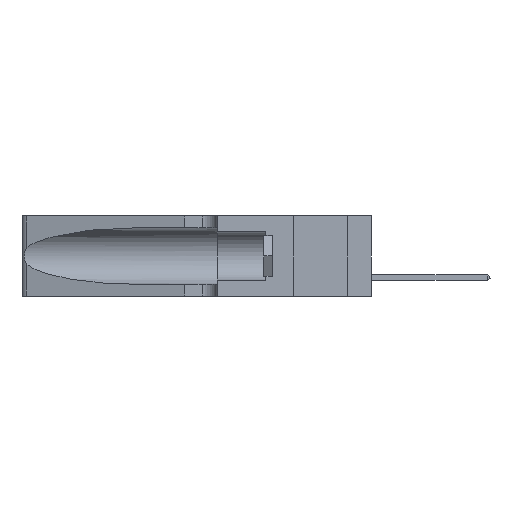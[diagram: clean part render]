
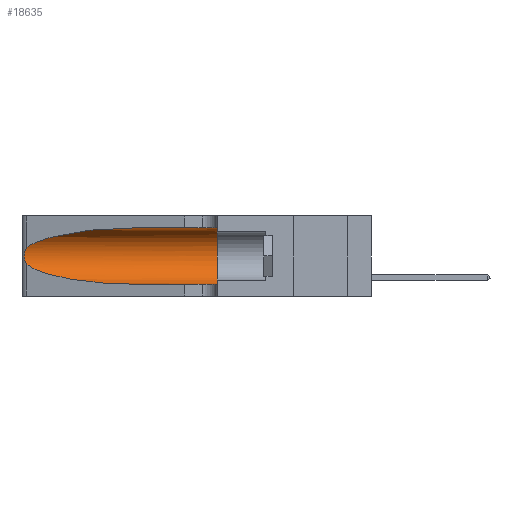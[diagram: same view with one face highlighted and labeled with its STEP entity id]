
A CAD part, left-side view. The second image highlights one B-rep face of the part: STEP entity #18635.
In plain terms, the highlighted cylindrical face has radius 3.308 mm (diameter 6.617 mm), a partial arc.
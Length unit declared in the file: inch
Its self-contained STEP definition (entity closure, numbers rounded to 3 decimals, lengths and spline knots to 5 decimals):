
#292 = DIRECTION ( 'NONE',  ( 0., 0., 1. ) ) ;
#557 = CARTESIAN_POINT ( 'NONE',  ( 0.26075, 1.23896, 0.19203 ) ) ;
#892 = DIRECTION ( 'NONE',  ( 0., -1., 0. ) ) ;
#2147 = VERTEX_POINT ( 'NONE', #2160 ) ;
#2160 = CARTESIAN_POINT ( 'NONE',  ( 0.1305, 0.35, 0.31525 ) ) ;
#2816 = VERTEX_POINT ( 'NONE', #16164 ) ;
#2926 = CIRCLE ( 'NONE', #32977, 0.13025 ) ;
#3227 = CARTESIAN_POINT ( 'NONE',  ( 0.25487, 1.22718, 0.14631 ) ) ;
#3683 = DIRECTION ( 'NONE',  ( 0., 1., 0. ) ) ;
#3934 = CARTESIAN_POINT ( 'NONE',  ( 0.26018, 1.23835, 0.19895 ) ) ;
#4049 = LINE ( 'NONE', #35554, #8653 ) ;
#6764 = ORIENTED_EDGE ( 'NONE', *, *, #40059, .F. ) ;
#6802 = B_SPLINE_CURVE_WITH_KNOTS ( 'NONE', 3,
 ( #33752, #18810, #18976, #15438, #41116, #3934, #557, #19125, #15267, #15605, #7940, #11276, #44798, #44950 ),
 .UNSPECIFIED., .F., .F.,
 ( 4, 2, 2, 2, 2, 2, 4 ),
 ( 0., 0.00027, 0.00053, 0.00107, 0.0016, 0.00187, 0.00214 ),
 .UNSPECIFIED. ) ;
#7940 = CARTESIAN_POINT ( 'NONE',  ( 0.25789, 1.23486, 0.15765 ) ) ;
#7962 = CARTESIAN_POINT ( 'NONE',  ( 0.1305, 1.61858, 0.31525 ) ) ;
#8653 = VECTOR ( 'NONE', #16770, 39.37008 ) ;
#11044 = CARTESIAN_POINT ( 'NONE',  ( 0.2373, 1.15595, 0.08982 ) ) ;
#11276 = CARTESIAN_POINT ( 'NONE',  ( 0.25639, 1.23186, 0.15144 ) ) ;
#13422 = DIRECTION ( 'NONE',  ( 0., 0., -1. ) ) ;
#14965 = CARTESIAN_POINT ( 'NONE',  ( 0.25487, 1.22718, 0.22369 ) ) ;
#15267 = CARTESIAN_POINT ( 'NONE',  ( 0.26017, 1.23833, 0.17102 ) ) ;
#15311 =( BOUNDED_CURVE ( )  B_SPLINE_CURVE ( 3, ( #25751, #32349, #43531, #14965 ),
 .UNSPECIFIED., .F., .F. ) 
 B_SPLINE_CURVE_WITH_KNOTS ( ( 4, 4 ),
 ( 1.5708, 2.84003 ),
 .UNSPECIFIED. ) 
 CURVE ( )  GEOMETRIC_REPRESENTATION_ITEM ( )  RATIONAL_B_SPLINE_CURVE ( ( 1., 0.87, 0.87, 1. ) ) 
 REPRESENTATION_ITEM ( '' )  );
#15438 = CARTESIAN_POINT ( 'NONE',  ( 0.25787, 1.23484, 0.2124 ) ) ;
#15444 = VECTOR ( 'NONE', #892, 39.37008 ) ;
#15605 = CARTESIAN_POINT ( 'NONE',  ( 0.25856, 1.23593, 0.16098 ) ) ;
#16164 = CARTESIAN_POINT ( 'NONE',  ( 0.1305, 0.72297, 0.05475 ) ) ;
#16770 = DIRECTION ( 'NONE',  ( 0., -1., 0. ) ) ;
#17588 = VERTEX_POINT ( 'NONE', #23264 ) ;
#18411 = CARTESIAN_POINT ( 'NONE',  ( 0.25487, 1.22718, 0.14631 ) ) ;
#18635 = ADVANCED_FACE ( 'NONE', ( #27746 ), #36898, .F. ) ;
#18810 = CARTESIAN_POINT ( 'NONE',  ( 0.25555, 1.22994, 0.2215 ) ) ;
#18976 = CARTESIAN_POINT ( 'NONE',  ( 0.25639, 1.23184, 0.21858 ) ) ;
#19125 = CARTESIAN_POINT ( 'NONE',  ( 0.26075, 1.23896, 0.178 ) ) ;
#19325 = ORIENTED_EDGE ( 'NONE', *, *, #38150, .T. ) ;
#20783 = CARTESIAN_POINT ( 'NONE',  ( 0.1305, 1.61858, 0.185 ) ) ;
#20936 = EDGE_CURVE ( 'NONE', #38564, #2147, #44719, .T. ) ;
#23264 = CARTESIAN_POINT ( 'NONE',  ( 0.25487, 1.22718, 0.22369 ) ) ;
#23599 = EDGE_CURVE ( 'NONE', #38564, #17588, #15311, .T. ) ;
#25751 = CARTESIAN_POINT ( 'NONE',  ( 0.1305, 0.72297, 0.31525 ) ) ;
#25974 = CARTESIAN_POINT ( 'NONE',  ( 0.1305, 0.35, 0.185 ) ) ;
#26212 = ORIENTED_EDGE ( 'NONE', *, *, #43004, .T. ) ;
#27746 = FACE_OUTER_BOUND ( 'NONE', #40491, .T. ) ;
#27956 = CARTESIAN_POINT ( 'NONE',  ( 0.1305, 0.35, 0.05475 ) ) ;
#29355 = CARTESIAN_POINT ( 'NONE',  ( 0.18966, 0.96281, 0.05475 ) ) ;
#30847 = ORIENTED_EDGE ( 'NONE', *, *, #23599, .T. ) ;
#31958 = CARTESIAN_POINT ( 'NONE',  ( 0.1305, 0.72297, 0.31525 ) ) ;
#32349 = CARTESIAN_POINT ( 'NONE',  ( 0.18966, 0.96281, 0.31525 ) ) ;
#32977 = AXIS2_PLACEMENT_3D ( 'NONE', #25974, #3683, #292 ) ;
#33752 = CARTESIAN_POINT ( 'NONE',  ( 0.25487, 1.22718, 0.22369 ) ) ;
#35554 = CARTESIAN_POINT ( 'NONE',  ( 0.1305, 1.61858, 0.05475 ) ) ;
#36460 = AXIS2_PLACEMENT_3D ( 'NONE', #20783, #39413, #13422 ) ;
#36718 = CARTESIAN_POINT ( 'NONE',  ( 0.1305, 0.72297, 0.05475 ) ) ;
#36898 = CYLINDRICAL_SURFACE ( 'NONE', #36460, 0.13025 ) ;
#38150 = EDGE_CURVE ( 'NONE', #17588, #38516, #6802, .T. ) ;
#38516 = VERTEX_POINT ( 'NONE', #3227 ) ;
#38564 = VERTEX_POINT ( 'NONE', #31958 ) ;
#38893 = ORIENTED_EDGE ( 'NONE', *, *, #20936, .F. ) ;
#39112 = VERTEX_POINT ( 'NONE', #27956 ) ;
#39413 = DIRECTION ( 'NONE',  ( 0., -1., 0. ) ) ;
#40059 = EDGE_CURVE ( 'NONE', #2147, #39112, #2926, .T. ) ;
#40289 = EDGE_CURVE ( 'NONE', #2816, #39112, #4049, .T. ) ;
#40491 = EDGE_LOOP ( 'NONE', ( #30847, #19325, #26212, #46946, #6764, #38893 ) ) ;
#41116 = CARTESIAN_POINT ( 'NONE',  ( 0.25854, 1.2359, 0.20912 ) ) ;
#41509 =( BOUNDED_CURVE ( )  B_SPLINE_CURVE ( 3, ( #18411, #11044, #29355, #36718 ),
 .UNSPECIFIED., .F., .F. ) 
 B_SPLINE_CURVE_WITH_KNOTS ( ( 4, 4 ),
 ( 3.44316, 4.71239 ),
 .UNSPECIFIED. ) 
 CURVE ( )  GEOMETRIC_REPRESENTATION_ITEM ( )  RATIONAL_B_SPLINE_CURVE ( ( 1., 0.87, 0.87, 1. ) ) 
 REPRESENTATION_ITEM ( '' )  );
#43004 = EDGE_CURVE ( 'NONE', #38516, #2816, #41509, .T. ) ;
#43531 = CARTESIAN_POINT ( 'NONE',  ( 0.2373, 1.15595, 0.28018 ) ) ;
#44719 = LINE ( 'NONE', #7962, #15444 ) ;
#44798 = CARTESIAN_POINT ( 'NONE',  ( 0.25555, 1.22993, 0.14849 ) ) ;
#44950 = CARTESIAN_POINT ( 'NONE',  ( 0.25487, 1.22718, 0.14631 ) ) ;
#46946 = ORIENTED_EDGE ( 'NONE', *, *, #40289, .T. ) ;
